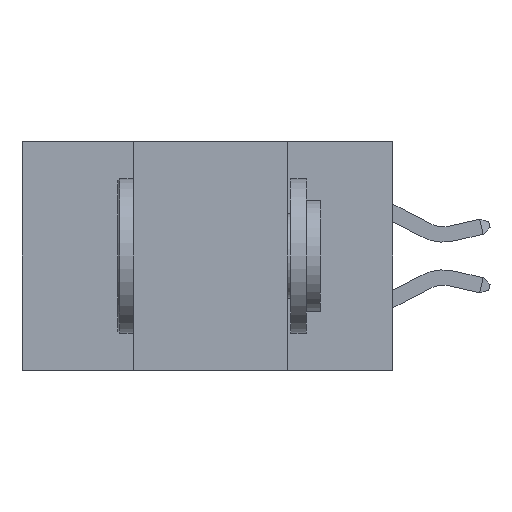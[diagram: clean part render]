
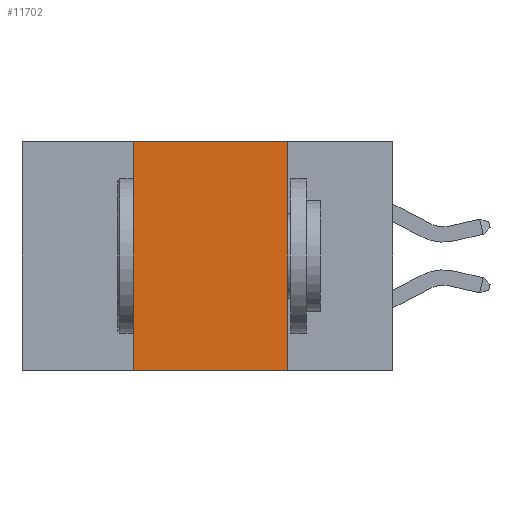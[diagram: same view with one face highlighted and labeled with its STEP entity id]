
A CAD part, left-side view. The second image highlights one B-rep face of the part: STEP entity #11702.
In plain terms, the highlighted planar face has unit normal (-1, 0, 0).
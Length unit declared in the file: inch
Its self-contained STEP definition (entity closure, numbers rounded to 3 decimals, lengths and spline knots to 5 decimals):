
#139 = CARTESIAN_POINT ( 'NONE',  ( 0., 0.17, 0. ) ) ;
#1363 = CARTESIAN_POINT ( 'NONE',  ( 0., 0.6, 0. ) ) ;
#1749 = FACE_OUTER_BOUND ( 'NONE', #31875, .T. ) ;
#2466 = ORIENTED_EDGE ( 'NONE', *, *, #8150, .F. ) ;
#2815 = VECTOR ( 'NONE', #21406, 39.37008 ) ;
#4097 = EDGE_CURVE ( 'NONE', #26820, #23582, #18803, .T. ) ;
#4133 = DIRECTION ( 'NONE',  ( 1., 0., 0. ) ) ;
#5140 = CARTESIAN_POINT ( 'NONE',  ( 0., 0.42, 0. ) ) ;
#5171 = VERTEX_POINT ( 'NONE', #13899 ) ;
#8150 = EDGE_CURVE ( 'NONE', #5171, #23582, #30659, .T. ) ;
#9915 = DIRECTION ( 'NONE',  ( 0., -1., 0. ) ) ;
#10605 = EDGE_CURVE ( 'NONE', #26820, #11572, #26130, .T. ) ;
#11572 = VERTEX_POINT ( 'NONE', #24580 ) ;
#11702 = ADVANCED_FACE ( 'NONE', ( #1749 ), #17311, .F. ) ;
#11859 = VECTOR ( 'NONE', #9915, 39.37008 ) ;
#12251 = AXIS2_PLACEMENT_3D ( 'NONE', #1363, #4133, #22563 ) ;
#13899 = CARTESIAN_POINT ( 'NONE',  ( 0., 0.17, 0. ) ) ;
#15370 = ORIENTED_EDGE ( 'NONE', *, *, #20827, .F. ) ;
#17311 = PLANE ( 'NONE',  #12251 ) ;
#17705 = CARTESIAN_POINT ( 'NONE',  ( 0., 0.6, -0.37 ) ) ;
#18803 = LINE ( 'NONE', #17705, #11859 ) ;
#20609 = LINE ( 'NONE', #30326, #25076 ) ;
#20827 = EDGE_CURVE ( 'NONE', #11572, #5171, #20609, .T. ) ;
#21406 = DIRECTION ( 'NONE',  ( 0., 0., -1. ) ) ;
#22177 = CARTESIAN_POINT ( 'NONE',  ( 0., 0.17, -0.37 ) ) ;
#22563 = DIRECTION ( 'NONE',  ( 0., 0., -1. ) ) ;
#23582 = VERTEX_POINT ( 'NONE', #22177 ) ;
#23942 = ORIENTED_EDGE ( 'NONE', *, *, #10605, .F. ) ;
#24580 = CARTESIAN_POINT ( 'NONE',  ( 0., 0.42, 0. ) ) ;
#25076 = VECTOR ( 'NONE', #25288, 39.37008 ) ;
#25288 = DIRECTION ( 'NONE',  ( 0., -1., 0. ) ) ;
#25773 = CARTESIAN_POINT ( 'NONE',  ( 0., 0.42, -0.37 ) ) ;
#26104 = DIRECTION ( 'NONE',  ( 0., 0., 1. ) ) ;
#26130 = LINE ( 'NONE', #5140, #32100 ) ;
#26820 = VERTEX_POINT ( 'NONE', #25773 ) ;
#30326 = CARTESIAN_POINT ( 'NONE',  ( 0., 0.6, 0. ) ) ;
#30366 = ORIENTED_EDGE ( 'NONE', *, *, #4097, .T. ) ;
#30659 = LINE ( 'NONE', #139, #2815 ) ;
#31875 = EDGE_LOOP ( 'NONE', ( #2466, #15370, #23942, #30366 ) ) ;
#32100 = VECTOR ( 'NONE', #26104, 39.37008 ) ;
